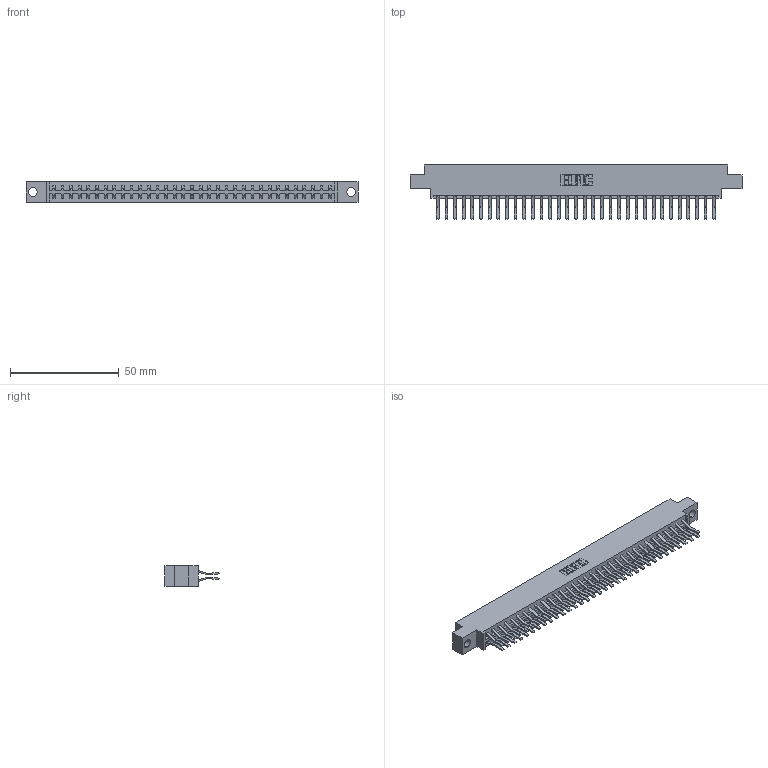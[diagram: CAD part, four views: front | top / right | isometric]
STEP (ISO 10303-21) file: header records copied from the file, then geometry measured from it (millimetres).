
FILE_DESCRIPTION (( 'STEP AP203' ), '1' );
FILE_NAME ('833-066-560-804.STEP', '2020-06-05T09:52:57', ( '' ), ( '' ), 'SwSTEP 2.0', 'SolidWorks 2020', '' );
FILE_SCHEMA (( 'CONFIG_CONTROL_DESIGN' ));
Length unit declared in the file: inch
Products named in the file (3): 833-066-560-804; 833 Part_Offset - .156 Dia - TH; 345-292-001_560 Tail
Assembly tree (67 placements, depth 2):
  833-066-560-804
    833 Part_Offset - .156 Dia - TH
    345-292-001_560 Tail  x66
Bounding box: 152.3 x 24.78 x 9.4 mm (x, y, z)
Volume: 15581.6 mm3; surface area: 19578.9 mm2
Topology: 67 solids, 67 shells, 3682 faces, 10949 edges, 7210 vertices
Faces by surface type: plane 2450, cylinder 1232
Entity records: 22617 total; most frequent: CARTESIAN_POINT 3762, ORIENTED_EDGE 3698, DIRECTION 3233, EDGE_CURVE 1849, VECTOR 1717, LINE 1717, VERTEX_POINT 1230, AXIS2_PLACEMENT_3D 758
